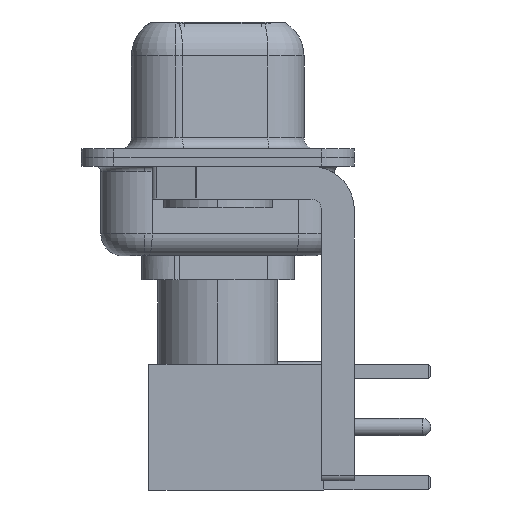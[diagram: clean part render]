
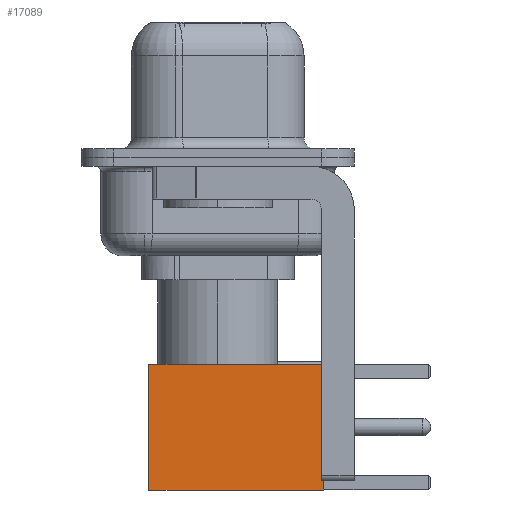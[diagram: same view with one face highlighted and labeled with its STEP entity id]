
A CAD part, left-side view. The second image highlights one B-rep face of the part: STEP entity #17089.
In plain terms, the highlighted face is planar.
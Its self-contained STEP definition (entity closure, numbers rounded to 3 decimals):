
#1503 = PLANE ( 'NONE',  #5911 ) ;
#2415 = VECTOR ( 'NONE', #20567, 1000. ) ;
#3180 = CARTESIAN_POINT ( 'NONE',  ( -2.875, 2.875, 0. ) ) ;
#3358 = CARTESIAN_POINT ( 'NONE',  ( 2.875, 2.875, 8. ) ) ;
#5507 = CARTESIAN_POINT ( 'NONE',  ( 2.875, 2.875, 0. ) ) ;
#5823 = CARTESIAN_POINT ( 'NONE',  ( 0., 2.875, 8. ) ) ;
#5911 = AXIS2_PLACEMENT_3D ( 'NONE', #22915, #19455, #8743 ) ;
#6549 = ORIENTED_EDGE ( 'NONE', *, *, #14275, .F. ) ;
#6705 = DIRECTION ( 'NONE',  ( -1., 0., 0. ) ) ;
#6816 = VERTEX_POINT ( 'NONE', #3358 ) ;
#6978 = CARTESIAN_POINT ( 'NONE',  ( -2.875, 2.875, 8. ) ) ;
#7657 = ORIENTED_EDGE ( 'NONE', *, *, #12582, .T. ) ;
#8071 = EDGE_CURVE ( 'NONE', #8825, #17166, #20413, .T. ) ;
#8743 = DIRECTION ( 'NONE',  ( 0., 0., 1. ) ) ;
#8825 = VERTEX_POINT ( 'NONE', #5507 ) ;
#11013 = VECTOR ( 'NONE', #6705, 1000. ) ;
#11381 = CARTESIAN_POINT ( 'NONE',  ( 0., 2.875, 0. ) ) ;
#11417 = DIRECTION ( 'NONE',  ( -1., 0., 0. ) ) ;
#12213 = FACE_OUTER_BOUND ( 'NONE', #21428, .T. ) ;
#12574 = EDGE_CURVE ( 'NONE', #6816, #14341, #18554, .T. ) ;
#12582 = EDGE_CURVE ( 'NONE', #6816, #8825, #21998, .T. ) ;
#13098 = CARTESIAN_POINT ( 'NONE',  ( 2.875, 2.875, 0. ) ) ;
#14097 = ORIENTED_EDGE ( 'NONE', *, *, #8071, .T. ) ;
#14275 = EDGE_CURVE ( 'NONE', #14341, #17166, #17352, .T. ) ;
#14341 = VERTEX_POINT ( 'NONE', #6978 ) ;
#15923 = DIRECTION ( 'NONE',  ( 0., 0., -1. ) ) ;
#17089 = ADVANCED_FACE ( 'NONE', ( #12213 ), #1503, .T. ) ;
#17166 = VERTEX_POINT ( 'NONE', #3180 ) ;
#17352 = LINE ( 'NONE', #17702, #21445 ) ;
#17702 = CARTESIAN_POINT ( 'NONE',  ( -2.875, 2.875, 0. ) ) ;
#18554 = LINE ( 'NONE', #5823, #22153 ) ;
#19455 = DIRECTION ( 'NONE',  ( 0., 1., 0. ) ) ;
#20413 = LINE ( 'NONE', #11381, #11013 ) ;
#20567 = DIRECTION ( 'NONE',  ( 0., 0., -1. ) ) ;
#20697 = ORIENTED_EDGE ( 'NONE', *, *, #12574, .F. ) ;
#21428 = EDGE_LOOP ( 'NONE', ( #7657, #14097, #6549, #20697 ) ) ;
#21445 = VECTOR ( 'NONE', #15923, 1000. ) ;
#21998 = LINE ( 'NONE', #13098, #2415 ) ;
#22153 = VECTOR ( 'NONE', #11417, 1000. ) ;
#22915 = CARTESIAN_POINT ( 'NONE',  ( 2.875, 2.875, 0. ) ) ;
